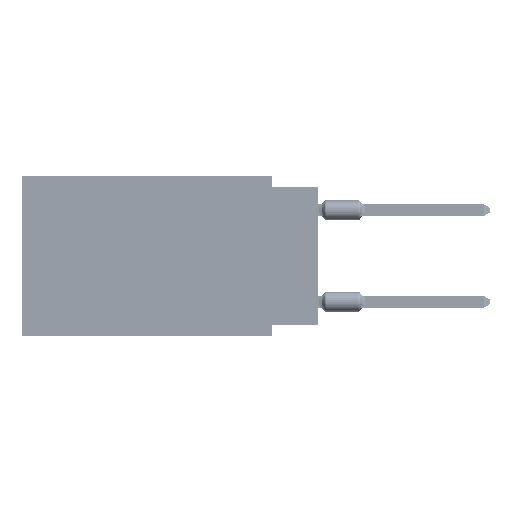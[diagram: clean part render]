
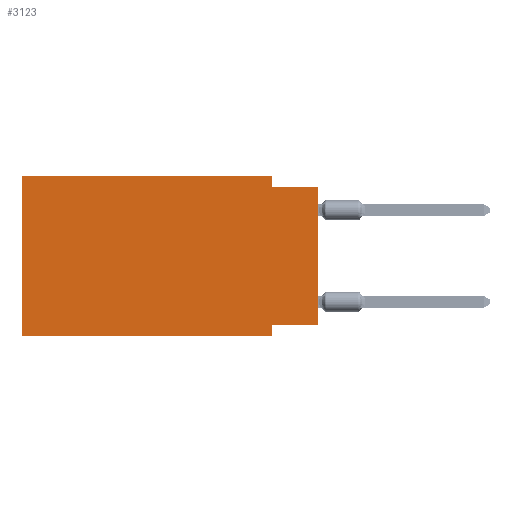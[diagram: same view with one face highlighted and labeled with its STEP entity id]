
A CAD part, left-side view. The second image highlights one B-rep face of the part: STEP entity #3123.
In plain terms, the highlighted planar face has unit normal (-1, 0, 0).
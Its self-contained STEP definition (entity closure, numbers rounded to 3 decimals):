
#246 = VERTEX_POINT ( 'NONE', #10477 ) ;
#3123 = ADVANCED_FACE ( 'NONE', ( #72352 ), #16679, .F. ) ;
#4541 = ORIENTED_EDGE ( 'NONE', *, *, #13260, .F. ) ;
#6095 = DIRECTION ( 'NONE',  ( 0., 0., 1. ) ) ;
#6570 = ORIENTED_EDGE ( 'NONE', *, *, #12251, .F. ) ;
#6628 = DIRECTION ( 'NONE',  ( 0., -1., 0. ) ) ;
#6988 = LINE ( 'NONE', #57661, #79940 ) ;
#7244 = VECTOR ( 'NONE', #27666, 1000. ) ;
#9895 = CARTESIAN_POINT ( 'NONE',  ( 0., 2.54, 0. ) ) ;
#10477 = CARTESIAN_POINT ( 'NONE',  ( 0., 2.54, -8.255 ) ) ;
#12251 = EDGE_CURVE ( 'NONE', #69971, #66669, #13057, .T. ) ;
#13057 = LINE ( 'NONE', #38192, #40069 ) ;
#13260 = EDGE_CURVE ( 'NONE', #66669, #43957, #28072, .T. ) ;
#13264 = VECTOR ( 'NONE', #63824, 1000. ) ;
#13392 = LINE ( 'NONE', #38934, #53658 ) ;
#13915 = CARTESIAN_POINT ( 'NONE',  ( 0., 16.383, -8.89 ) ) ;
#14505 = ORIENTED_EDGE ( 'NONE', *, *, #72215, .F. ) ;
#16327 = VERTEX_POINT ( 'NONE', #57742 ) ;
#16679 = PLANE ( 'NONE',  #43512 ) ;
#19315 = CARTESIAN_POINT ( 'NONE',  ( 0., 0., -8.255 ) ) ;
#27010 = EDGE_CURVE ( 'NONE', #77518, #16327, #74541, .T. ) ;
#27666 = DIRECTION ( 'NONE',  ( 0., 0., -1. ) ) ;
#28072 = LINE ( 'NONE', #48960, #7244 ) ;
#29956 = EDGE_CURVE ( 'NONE', #43957, #16327, #6988, .T. ) ;
#30983 = CARTESIAN_POINT ( 'NONE',  ( 0., 16.383, -8.89 ) ) ;
#31559 = DIRECTION ( 'NONE',  ( 0., 0., -1. ) ) ;
#31953 = CARTESIAN_POINT ( 'NONE',  ( 0., 2.54, -8.89 ) ) ;
#31989 = EDGE_CURVE ( 'NONE', #246, #70608, #13392, .T. ) ;
#32122 = ORIENTED_EDGE ( 'NONE', *, *, #35801, .F. ) ;
#35801 = EDGE_CURVE ( 'NONE', #77518, #246, #38683, .T. ) ;
#37153 = LINE ( 'NONE', #30983, #68951 ) ;
#37681 = ORIENTED_EDGE ( 'NONE', *, *, #29956, .F. ) ;
#38192 = CARTESIAN_POINT ( 'NONE',  ( 0., 16.383, 0. ) ) ;
#38683 = LINE ( 'NONE', #19315, #13264 ) ;
#38934 = CARTESIAN_POINT ( 'NONE',  ( 0., 2.54, -8.89 ) ) ;
#40069 = VECTOR ( 'NONE', #55143, 1000. ) ;
#43512 = AXIS2_PLACEMENT_3D ( 'NONE', #59964, #65745, #66566 ) ;
#43957 = VERTEX_POINT ( 'NONE', #73295 ) ;
#44590 = LINE ( 'NONE', #51596, #46755 ) ;
#46755 = VECTOR ( 'NONE', #70146, 1000. ) ;
#48960 = CARTESIAN_POINT ( 'NONE',  ( 0., 2.54, 0. ) ) ;
#50284 = DIRECTION ( 'NONE',  ( 0., -1., 0. ) ) ;
#50300 = ORIENTED_EDGE ( 'NONE', *, *, #31989, .F. ) ;
#50596 = CARTESIAN_POINT ( 'NONE',  ( 0., 0., 0. ) ) ;
#51540 = CARTESIAN_POINT ( 'NONE',  ( 0., 16.383, 0. ) ) ;
#51596 = CARTESIAN_POINT ( 'NONE',  ( 0., 16.383, 0. ) ) ;
#53658 = VECTOR ( 'NONE', #31559, 1000. ) ;
#55113 = CARTESIAN_POINT ( 'NONE',  ( 0., 0., -8.255 ) ) ;
#55143 = DIRECTION ( 'NONE',  ( 0., -1., 0. ) ) ;
#57661 = CARTESIAN_POINT ( 'NONE',  ( 0., 0., -0.635 ) ) ;
#57742 = CARTESIAN_POINT ( 'NONE',  ( 0., 0., -0.635 ) ) ;
#59964 = CARTESIAN_POINT ( 'NONE',  ( 0., 16.383, 0. ) ) ;
#63824 = DIRECTION ( 'NONE',  ( 0., 1., 0. ) ) ;
#65745 = DIRECTION ( 'NONE',  ( 1., 0., 0. ) ) ;
#66566 = DIRECTION ( 'NONE',  ( 0., 0., -1. ) ) ;
#66669 = VERTEX_POINT ( 'NONE', #9895 ) ;
#66933 = EDGE_LOOP ( 'NONE', ( #76665, #37681, #4541, #6570, #14505, #80094, #50300, #32122 ) ) ;
#68951 = VECTOR ( 'NONE', #6628, 1000. ) ;
#69106 = VERTEX_POINT ( 'NONE', #13915 ) ;
#69901 = EDGE_CURVE ( 'NONE', #69106, #70608, #37153, .T. ) ;
#69971 = VERTEX_POINT ( 'NONE', #51540 ) ;
#70146 = DIRECTION ( 'NONE',  ( 0., 0., 1. ) ) ;
#70608 = VERTEX_POINT ( 'NONE', #31953 ) ;
#72215 = EDGE_CURVE ( 'NONE', #69106, #69971, #44590, .T. ) ;
#72352 = FACE_OUTER_BOUND ( 'NONE', #66933, .T. ) ;
#73295 = CARTESIAN_POINT ( 'NONE',  ( 0., 2.54, -0.635 ) ) ;
#74541 = LINE ( 'NONE', #50596, #76997 ) ;
#76665 = ORIENTED_EDGE ( 'NONE', *, *, #27010, .T. ) ;
#76997 = VECTOR ( 'NONE', #6095, 1000. ) ;
#77518 = VERTEX_POINT ( 'NONE', #55113 ) ;
#79940 = VECTOR ( 'NONE', #50284, 1000. ) ;
#80094 = ORIENTED_EDGE ( 'NONE', *, *, #69901, .T. ) ;
